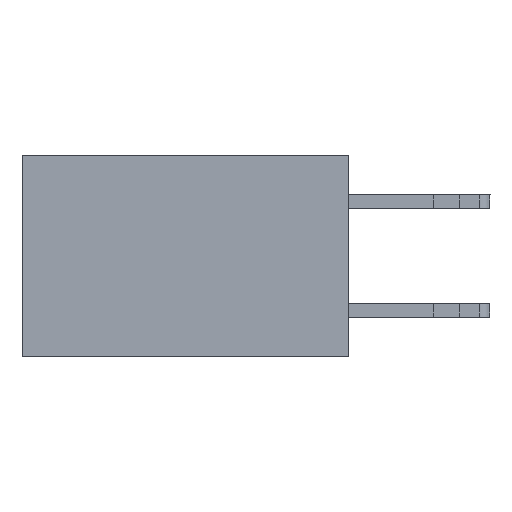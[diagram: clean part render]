
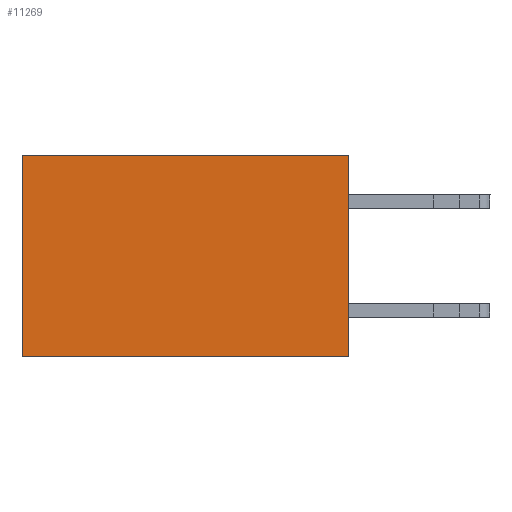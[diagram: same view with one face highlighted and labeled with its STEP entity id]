
A CAD part, left-side view. The second image highlights one B-rep face of the part: STEP entity #11269.
In plain terms, the highlighted planar face has unit normal (-1, 0, 0).
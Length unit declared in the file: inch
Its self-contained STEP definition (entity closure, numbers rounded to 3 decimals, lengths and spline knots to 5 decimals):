
#390 = CARTESIAN_POINT ( 'NONE',  ( 0.298, 0.6, -0.37 ) ) ;
#734 = DIRECTION ( 'NONE',  ( 1., 0., 0. ) ) ;
#917 = ORIENTED_EDGE ( 'NONE', *, *, #19750, .F. ) ;
#1815 = CARTESIAN_POINT ( 'NONE',  ( 0.298, 0.6, 0. ) ) ;
#1914 = ORIENTED_EDGE ( 'NONE', *, *, #25394, .F. ) ;
#3532 = LINE ( 'NONE', #5703, #21900 ) ;
#3747 = CARTESIAN_POINT ( 'NONE',  ( 0.298, 0., 0. ) ) ;
#4565 = VECTOR ( 'NONE', #20091, 39.37008 ) ;
#5089 = CARTESIAN_POINT ( 'NONE',  ( 0.298, 0., 0. ) ) ;
#5227 = FACE_OUTER_BOUND ( 'NONE', #18384, .T. ) ;
#5703 = CARTESIAN_POINT ( 'NONE',  ( 0.298, 0., -0.37 ) ) ;
#7200 = CARTESIAN_POINT ( 'NONE',  ( 0.298, 0., 0. ) ) ;
#8971 = VERTEX_POINT ( 'NONE', #13438 ) ;
#9094 = VERTEX_POINT ( 'NONE', #1815 ) ;
#9108 = ORIENTED_EDGE ( 'NONE', *, *, #24028, .T. ) ;
#9252 = LINE ( 'NONE', #7200, #23369 ) ;
#9388 = DIRECTION ( 'NONE',  ( 0., 1., 0. ) ) ;
#9391 = LINE ( 'NONE', #11446, #4565 ) ;
#11269 = ADVANCED_FACE ( 'NONE', ( #5227 ), #21958, .F. ) ;
#11446 = CARTESIAN_POINT ( 'NONE',  ( 0.298, 0., 0. ) ) ;
#13438 = CARTESIAN_POINT ( 'NONE',  ( 0.298, 0., -0.37 ) ) ;
#13485 = DIRECTION ( 'NONE',  ( 0., 0., -1. ) ) ;
#16376 = DIRECTION ( 'NONE',  ( 0., 1., 0. ) ) ;
#16907 = VERTEX_POINT ( 'NONE', #390 ) ;
#17338 = CARTESIAN_POINT ( 'NONE',  ( 0.298, 0.6, 0. ) ) ;
#18384 = EDGE_LOOP ( 'NONE', ( #22779, #917, #1914, #9108 ) ) ;
#18871 = VECTOR ( 'NONE', #13485, 39.37008 ) ;
#19750 = EDGE_CURVE ( 'NONE', #8971, #16907, #3532, .T. ) ;
#19805 = LINE ( 'NONE', #17338, #18871 ) ;
#20091 = DIRECTION ( 'NONE',  ( 0., 0., -1. ) ) ;
#21273 = EDGE_CURVE ( 'NONE', #9094, #16907, #19805, .T. ) ;
#21900 = VECTOR ( 'NONE', #16376, 39.37008 ) ;
#21958 = PLANE ( 'NONE',  #26801 ) ;
#22779 = ORIENTED_EDGE ( 'NONE', *, *, #21273, .T. ) ;
#23369 = VECTOR ( 'NONE', #9388, 39.37008 ) ;
#23613 = DIRECTION ( 'NONE',  ( 0., 0., -1. ) ) ;
#24028 = EDGE_CURVE ( 'NONE', #26023, #9094, #9252, .T. ) ;
#25394 = EDGE_CURVE ( 'NONE', #26023, #8971, #9391, .T. ) ;
#26023 = VERTEX_POINT ( 'NONE', #3747 ) ;
#26801 = AXIS2_PLACEMENT_3D ( 'NONE', #5089, #734, #23613 ) ;
